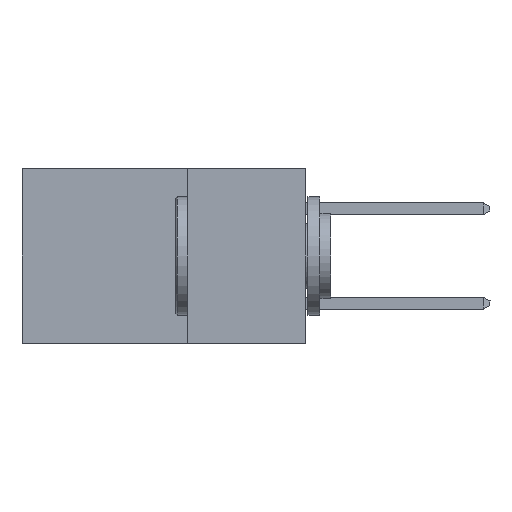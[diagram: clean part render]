
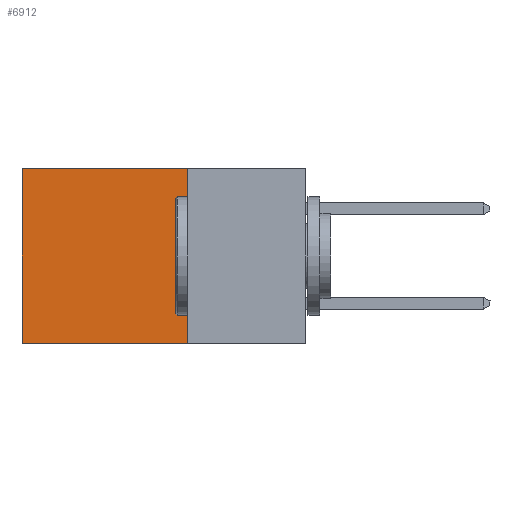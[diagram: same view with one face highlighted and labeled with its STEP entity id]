
A CAD part, left-side view. The second image highlights one B-rep face of the part: STEP entity #6912.
In plain terms, the highlighted planar face has unit normal (-1, 0, 0).
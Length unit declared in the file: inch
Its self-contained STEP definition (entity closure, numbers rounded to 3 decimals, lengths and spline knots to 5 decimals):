
#285 = VECTOR ( 'NONE', #5665, 39.37008 ) ;
#1282 = VECTOR ( 'NONE', #10165, 39.37008 ) ;
#1934 = CARTESIAN_POINT ( 'NONE',  ( 0.298, 0.25, -0.37 ) ) ;
#1994 = VECTOR ( 'NONE', #7309, 39.37008 ) ;
#2695 = VERTEX_POINT ( 'NONE', #2865 ) ;
#2706 = ORIENTED_EDGE ( 'NONE', *, *, #9124, .T. ) ;
#2767 = EDGE_CURVE ( 'NONE', #2695, #15600, #11208, .T. ) ;
#2865 = CARTESIAN_POINT ( 'NONE',  ( 0.298, 0.25, 0. ) ) ;
#3217 = CARTESIAN_POINT ( 'NONE',  ( 0.298, 0.25, 0. ) ) ;
#3521 = ORIENTED_EDGE ( 'NONE', *, *, #2767, .T. ) ;
#3527 = FACE_OUTER_BOUND ( 'NONE', #12095, .T. ) ;
#3637 = DIRECTION ( 'NONE',  ( 1., 0., 0. ) ) ;
#3760 = PLANE ( 'NONE',  #4253 ) ;
#4253 = AXIS2_PLACEMENT_3D ( 'NONE', #14169, #3637, #6209 ) ;
#4574 = VECTOR ( 'NONE', #4777, 39.37008 ) ;
#4747 = ORIENTED_EDGE ( 'NONE', *, *, #5101, .F. ) ;
#4777 = DIRECTION ( 'NONE',  ( 0., 1., 0. ) ) ;
#5059 = VERTEX_POINT ( 'NONE', #13982 ) ;
#5101 = EDGE_CURVE ( 'NONE', #5059, #7244, #6186, .T. ) ;
#5479 = LINE ( 'NONE', #15436, #1994 ) ;
#5665 = DIRECTION ( 'NONE',  ( 0., 1., 0. ) ) ;
#6186 = LINE ( 'NONE', #1934, #4574 ) ;
#6195 = CARTESIAN_POINT ( 'NONE',  ( 0.298, 0.6, 0. ) ) ;
#6202 = CARTESIAN_POINT ( 'NONE',  ( 0.298, 0.6, 0. ) ) ;
#6209 = DIRECTION ( 'NONE',  ( 0., 0., -1. ) ) ;
#6912 = ADVANCED_FACE ( 'NONE', ( #3527 ), #3760, .F. ) ;
#7244 = VERTEX_POINT ( 'NONE', #17072 ) ;
#7309 = DIRECTION ( 'NONE',  ( 0., 0., -1. ) ) ;
#9124 = EDGE_CURVE ( 'NONE', #15600, #7244, #13689, .T. ) ;
#10165 = DIRECTION ( 'NONE',  ( 0., 0., -1. ) ) ;
#11208 = LINE ( 'NONE', #3217, #285 ) ;
#11912 = EDGE_CURVE ( 'NONE', #2695, #5059, #5479, .T. ) ;
#12095 = EDGE_LOOP ( 'NONE', ( #2706, #4747, #13701, #3521 ) ) ;
#13689 = LINE ( 'NONE', #6202, #1282 ) ;
#13701 = ORIENTED_EDGE ( 'NONE', *, *, #11912, .F. ) ;
#13982 = CARTESIAN_POINT ( 'NONE',  ( 0.298, 0.25, -0.37 ) ) ;
#14169 = CARTESIAN_POINT ( 'NONE',  ( 0.298, 0.25, 0. ) ) ;
#15436 = CARTESIAN_POINT ( 'NONE',  ( 0.298, 0.25, 0. ) ) ;
#15600 = VERTEX_POINT ( 'NONE', #6195 ) ;
#17072 = CARTESIAN_POINT ( 'NONE',  ( 0.298, 0.6, -0.37 ) ) ;
